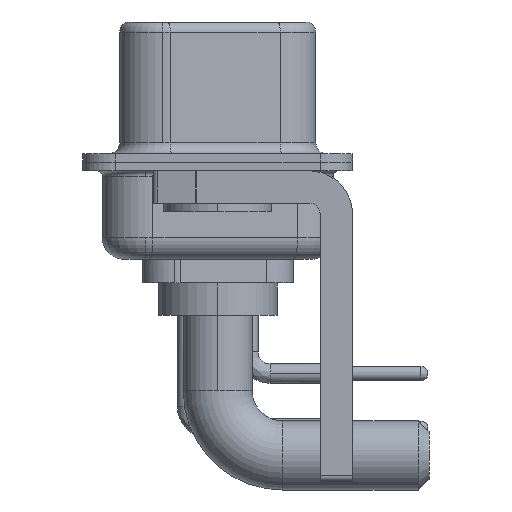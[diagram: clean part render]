
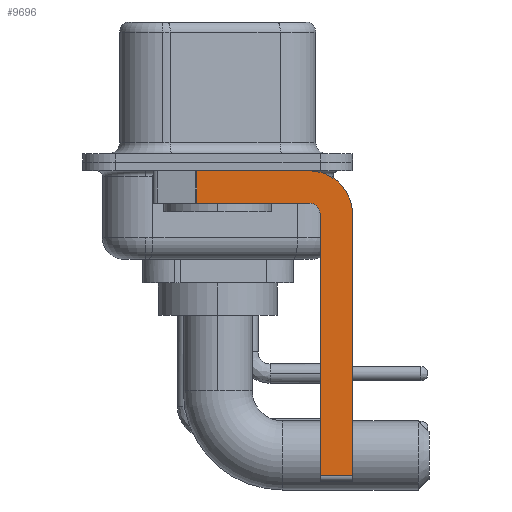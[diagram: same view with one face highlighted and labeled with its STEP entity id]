
A CAD part, left-side view. The second image highlights one B-rep face of the part: STEP entity #9696.
In plain terms, the highlighted planar face has unit normal (-1, 0, 0).
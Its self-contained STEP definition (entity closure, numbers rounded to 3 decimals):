
#381 = VERTEX_POINT ( 'NONE', #14279 ) ;
#438 = VECTOR ( 'NONE', #21194, 1000. ) ;
#1211 = VERTEX_POINT ( 'NONE', #13671 ) ;
#1231 = CARTESIAN_POINT ( 'NONE',  ( -2.9, -4.75, -2.4 ) ) ;
#2543 = ORIENTED_EDGE ( 'NONE', *, *, #4746, .F. ) ;
#2779 = LINE ( 'NONE', #10283, #12432 ) ;
#2862 = ORIENTED_EDGE ( 'NONE', *, *, #9016, .F. ) ;
#3084 = EDGE_CURVE ( 'NONE', #13440, #1211, #8149, .T. ) ;
#3132 = LINE ( 'NONE', #24925, #12058 ) ;
#3652 = VERTEX_POINT ( 'NONE', #1231 ) ;
#3798 = FACE_OUTER_BOUND ( 'NONE', #19731, .T. ) ;
#4715 = CARTESIAN_POINT ( 'NONE',  ( -2.9, -4.25, -2.4 ) ) ;
#4746 = EDGE_CURVE ( 'NONE', #13440, #3652, #7511, .T. ) ;
#5581 = CARTESIAN_POINT ( 'NONE',  ( -2.9, -4.75, -14.8 ) ) ;
#6535 = CARTESIAN_POINT ( 'NONE',  ( -2.9, -4.25, -2.4 ) ) ;
#7149 = CARTESIAN_POINT ( 'NONE',  ( -2.9, 0.978, -0.4 ) ) ;
#7268 = DIRECTION ( 'NONE',  ( 0., 0., -1. ) ) ;
#7511 = LINE ( 'NONE', #5581, #438 ) ;
#7512 = LINE ( 'NONE', #17313, #21902 ) ;
#8017 = DIRECTION ( 'NONE',  ( 0., -1., 0. ) ) ;
#8149 = LINE ( 'NONE', #19880, #24053 ) ;
#9016 = EDGE_CURVE ( 'NONE', #20243, #21563, #7512, .T. ) ;
#9314 = VERTEX_POINT ( 'NONE', #14583 ) ;
#9530 = ORIENTED_EDGE ( 'NONE', *, *, #11286, .F. ) ;
#9696 = ADVANCED_FACE ( 'NONE', ( #3798 ), #17609, .F. ) ;
#9745 = CARTESIAN_POINT ( 'NONE',  ( -2.9, -4.75, -14.55 ) ) ;
#10245 = DIRECTION ( 'NONE',  ( 1., 0., 0. ) ) ;
#10283 = CARTESIAN_POINT ( 'NONE',  ( -2.9, -4.25, -1.9 ) ) ;
#10780 = DIRECTION ( 'NONE',  ( 0., 0., -1. ) ) ;
#11286 = EDGE_CURVE ( 'NONE', #20162, #1211, #3132, .T. ) ;
#11599 = ORIENTED_EDGE ( 'NONE', *, *, #3084, .T. ) ;
#12058 = VECTOR ( 'NONE', #7268, 1000. ) ;
#12432 = VECTOR ( 'NONE', #23943, 1000. ) ;
#12729 = DIRECTION ( 'NONE',  ( 1., 0., 0. ) ) ;
#13440 = VERTEX_POINT ( 'NONE', #9745 ) ;
#13671 = CARTESIAN_POINT ( 'NONE',  ( -2.9, -6.25, -14.55 ) ) ;
#13749 = CARTESIAN_POINT ( 'NONE',  ( -2.9, -4.25, -2.4 ) ) ;
#14279 = CARTESIAN_POINT ( 'NONE',  ( -2.9, -4.25, -1.9 ) ) ;
#14427 = ORIENTED_EDGE ( 'NONE', *, *, #18910, .F. ) ;
#14583 = CARTESIAN_POINT ( 'NONE',  ( -2.9, 0.978, -1.9 ) ) ;
#14662 = DIRECTION ( 'NONE',  ( 0., 0., 1. ) ) ;
#15008 = DIRECTION ( 'NONE',  ( 0., 0., -1. ) ) ;
#15306 = AXIS2_PLACEMENT_3D ( 'NONE', #6535, #22263, #14662 ) ;
#15562 = DIRECTION ( 'NONE',  ( 0., 0., -1. ) ) ;
#15774 = ORIENTED_EDGE ( 'NONE', *, *, #16017, .T. ) ;
#15921 = VECTOR ( 'NONE', #15008, 1000. ) ;
#16017 = EDGE_CURVE ( 'NONE', #20243, #9314, #20425, .T. ) ;
#16476 = AXIS2_PLACEMENT_3D ( 'NONE', #4715, #12729, #10780 ) ;
#17313 = CARTESIAN_POINT ( 'NONE',  ( -2.9, 3., -0.4 ) ) ;
#17447 = DIRECTION ( 'NONE',  ( 0., -1., 0. ) ) ;
#17609 = PLANE ( 'NONE',  #18209 ) ;
#18209 = AXIS2_PLACEMENT_3D ( 'NONE', #13749, #10245, #15562 ) ;
#18601 = CIRCLE ( 'NONE', #15306, 0.5 ) ;
#18910 = EDGE_CURVE ( 'NONE', #21563, #20162, #23866, .T. ) ;
#19653 = EDGE_CURVE ( 'NONE', #381, #9314, #2779, .T. ) ;
#19690 = EDGE_CURVE ( 'NONE', #3652, #381, #18601, .T. ) ;
#19731 = EDGE_LOOP ( 'NONE', ( #2862, #15774, #20468, #23160, #2543, #11599, #9530, #14427 ) ) ;
#19880 = CARTESIAN_POINT ( 'NONE',  ( -2.9, -4.25, -14.55 ) ) ;
#20162 = VERTEX_POINT ( 'NONE', #22878 ) ;
#20243 = VERTEX_POINT ( 'NONE', #7149 ) ;
#20315 = CARTESIAN_POINT ( 'NONE',  ( -2.9, -4.25, -0.4 ) ) ;
#20425 = LINE ( 'NONE', #24781, #15921 ) ;
#20468 = ORIENTED_EDGE ( 'NONE', *, *, #19653, .F. ) ;
#21194 = DIRECTION ( 'NONE',  ( 0., 0., 1. ) ) ;
#21563 = VERTEX_POINT ( 'NONE', #20315 ) ;
#21902 = VECTOR ( 'NONE', #17447, 1000. ) ;
#22263 = DIRECTION ( 'NONE',  ( -1., 0., 0. ) ) ;
#22878 = CARTESIAN_POINT ( 'NONE',  ( -2.9, -6.25, -2.4 ) ) ;
#23160 = ORIENTED_EDGE ( 'NONE', *, *, #19690, .F. ) ;
#23866 = CIRCLE ( 'NONE', #16476, 2. ) ;
#23943 = DIRECTION ( 'NONE',  ( 0., 1., 0. ) ) ;
#24053 = VECTOR ( 'NONE', #8017, 1000. ) ;
#24781 = CARTESIAN_POINT ( 'NONE',  ( -2.9, 0.978, -1.9 ) ) ;
#24925 = CARTESIAN_POINT ( 'NONE',  ( -2.9, -6.25, -2.4 ) ) ;
